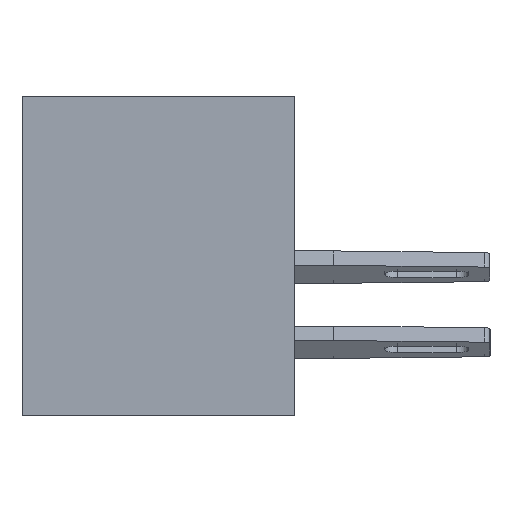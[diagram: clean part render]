
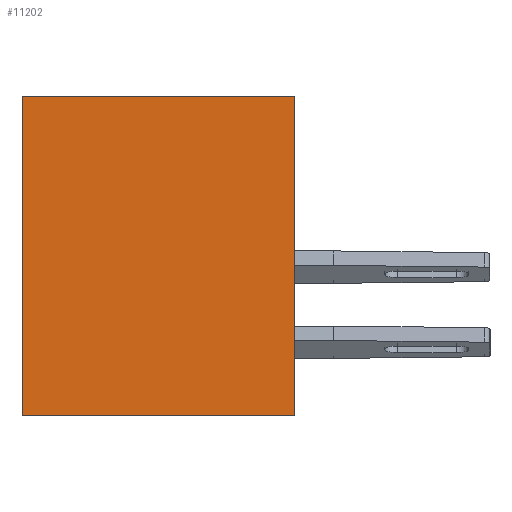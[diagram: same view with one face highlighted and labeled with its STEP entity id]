
A CAD part, left-side view. The second image highlights one B-rep face of the part: STEP entity #11202.
In plain terms, the highlighted planar face has unit normal (-1, 0, 0).
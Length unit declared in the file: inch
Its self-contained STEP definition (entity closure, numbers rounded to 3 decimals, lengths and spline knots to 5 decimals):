
#394 = EDGE_LOOP ( 'NONE', ( #12210, #21939, #27336, #14425 ) ) ;
#2207 = EDGE_CURVE ( 'NONE', #4360, #18746, #19299, .T. ) ;
#3869 = CARTESIAN_POINT ( 'NONE',  ( 0., 0.453, -0.531 ) ) ;
#4106 = CARTESIAN_POINT ( 'NONE',  ( 0., 0.453, 0. ) ) ;
#4360 = VERTEX_POINT ( 'NONE', #4106 ) ;
#4432 = LINE ( 'NONE', #16064, #15395 ) ;
#5933 = DIRECTION ( 'NONE',  ( 0., 0., -1. ) ) ;
#7767 = EDGE_CURVE ( 'NONE', #27470, #4360, #22558, .T. ) ;
#9546 = CARTESIAN_POINT ( 'NONE',  ( 0., 0., -0.531 ) ) ;
#11202 = ADVANCED_FACE ( 'NONE', ( #11336 ), #18873, .F. ) ;
#11336 = FACE_OUTER_BOUND ( 'NONE', #394, .T. ) ;
#11594 = EDGE_CURVE ( 'NONE', #27470, #14901, #18043, .T. ) ;
#12210 = ORIENTED_EDGE ( 'NONE', *, *, #27161, .T. ) ;
#13043 = DIRECTION ( 'NONE',  ( 0., -1., 0. ) ) ;
#14425 = ORIENTED_EDGE ( 'NONE', *, *, #11594, .T. ) ;
#14901 = VERTEX_POINT ( 'NONE', #9546 ) ;
#15266 = CARTESIAN_POINT ( 'NONE',  ( 0., 0., 0. ) ) ;
#15395 = VECTOR ( 'NONE', #18200, 39.37008 ) ;
#16064 = CARTESIAN_POINT ( 'NONE',  ( 0., 0., 0. ) ) ;
#16972 = CARTESIAN_POINT ( 'NONE',  ( 0., 0.453, -0.531 ) ) ;
#18043 = LINE ( 'NONE', #3869, #21031 ) ;
#18200 = DIRECTION ( 'NONE',  ( 0., 0., 1. ) ) ;
#18746 = VERTEX_POINT ( 'NONE', #15266 ) ;
#18873 = PLANE ( 'NONE',  #25852 ) ;
#19299 = LINE ( 'NONE', #23646, #25966 ) ;
#20912 = CARTESIAN_POINT ( 'NONE',  ( 0., 0.453, 0. ) ) ;
#21031 = VECTOR ( 'NONE', #25266, 39.37008 ) ;
#21850 = DIRECTION ( 'NONE',  ( 0., 0., 1. ) ) ;
#21939 = ORIENTED_EDGE ( 'NONE', *, *, #2207, .F. ) ;
#22558 = LINE ( 'NONE', #23887, #26912 ) ;
#23646 = CARTESIAN_POINT ( 'NONE',  ( 0., 0.453, 0. ) ) ;
#23887 = CARTESIAN_POINT ( 'NONE',  ( 0., 0.453, 0. ) ) ;
#25190 = DIRECTION ( 'NONE',  ( 1., 0., 0. ) ) ;
#25266 = DIRECTION ( 'NONE',  ( 0., -1., 0. ) ) ;
#25852 = AXIS2_PLACEMENT_3D ( 'NONE', #20912, #25190, #5933 ) ;
#25966 = VECTOR ( 'NONE', #13043, 39.37008 ) ;
#26912 = VECTOR ( 'NONE', #21850, 39.37008 ) ;
#27161 = EDGE_CURVE ( 'NONE', #14901, #18746, #4432, .T. ) ;
#27336 = ORIENTED_EDGE ( 'NONE', *, *, #7767, .F. ) ;
#27470 = VERTEX_POINT ( 'NONE', #16972 ) ;
